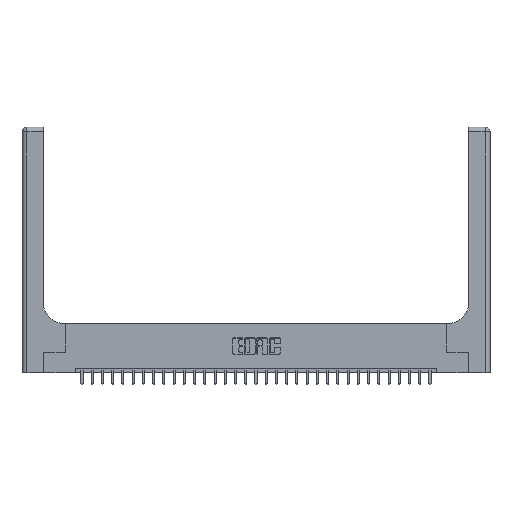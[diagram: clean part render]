
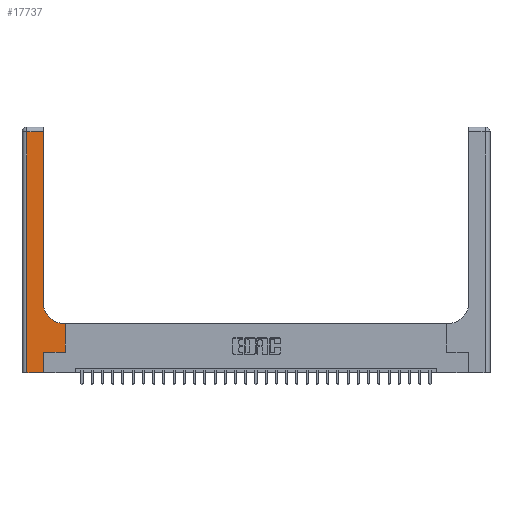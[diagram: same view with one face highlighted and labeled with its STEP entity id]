
A CAD part, top view. The second image highlights one B-rep face of the part: STEP entity #17737.
In plain terms, the highlighted planar face has unit normal (0, 0, 1).
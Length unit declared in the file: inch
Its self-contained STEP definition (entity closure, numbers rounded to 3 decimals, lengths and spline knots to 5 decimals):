
#203 = DIRECTION ( 'NONE',  ( 0., 0., -1. ) ) ;
#1018 = ORIENTED_EDGE ( 'NONE', *, *, #15994, .T. ) ;
#1087 = DIRECTION ( 'NONE',  ( 0., 1., 0. ) ) ;
#2089 = LINE ( 'NONE', #12986, #9763 ) ;
#2160 = EDGE_CURVE ( 'NONE', #9387, #17589, #18202, .T. ) ;
#2320 = ORIENTED_EDGE ( 'NONE', *, *, #22164, .T. ) ;
#2910 = CARTESIAN_POINT ( 'NONE',  ( 0.528, 0.6, 0.37 ) ) ;
#2916 = AXIS2_PLACEMENT_3D ( 'NONE', #20923, #203, #11976 ) ;
#2946 = CIRCLE ( 'NONE', #22953, 0.25 ) ;
#3421 = EDGE_CURVE ( 'NONE', #23773, #5509, #5814, .T. ) ;
#3538 = LINE ( 'NONE', #25630, #8011 ) ;
#3677 = VERTEX_POINT ( 'NONE', #5182 ) ;
#3708 = CARTESIAN_POINT ( 'NONE',  ( 0.528, 0.25, 0.37 ) ) ;
#4379 = CARTESIAN_POINT ( 'NONE',  ( 0.265, 0., 0.37 ) ) ;
#4380 = ORIENTED_EDGE ( 'NONE', *, *, #15150, .T. ) ;
#4567 = VERTEX_POINT ( 'NONE', #17945 ) ;
#4913 = DIRECTION ( 'NONE',  ( 1., 0., 0. ) ) ;
#5182 = CARTESIAN_POINT ( 'NONE',  ( 0.06, 2.94, 0.37 ) ) ;
#5497 = EDGE_CURVE ( 'NONE', #3677, #9387, #7105, .T. ) ;
#5509 = VERTEX_POINT ( 'NONE', #2910 ) ;
#5814 = LINE ( 'NONE', #3708, #28972 ) ;
#5893 = ORIENTED_EDGE ( 'NONE', *, *, #2160, .T. ) ;
#6213 = LINE ( 'NONE', #6357, #26730 ) ;
#6357 = CARTESIAN_POINT ( 'NONE',  ( 0., 2.94, 0.37 ) ) ;
#7105 = LINE ( 'NONE', #13254, #16096 ) ;
#7249 = DIRECTION ( 'NONE',  ( 0., -1., 0. ) ) ;
#7363 = CARTESIAN_POINT ( 'NONE',  ( 0.528, 0.25, 0.37 ) ) ;
#8011 = VECTOR ( 'NONE', #28156, 39.37008 ) ;
#8025 = EDGE_CURVE ( 'NONE', #17589, #13931, #14653, .T. ) ;
#8221 = CARTESIAN_POINT ( 'NONE',  ( 0.26, 0.85, 0.37 ) ) ;
#8770 = ORIENTED_EDGE ( 'NONE', *, *, #25700, .T. ) ;
#9369 = ORIENTED_EDGE ( 'NONE', *, *, #5497, .T. ) ;
#9387 = VERTEX_POINT ( 'NONE', #14657 ) ;
#9763 = VECTOR ( 'NONE', #26718, 39.37008 ) ;
#10508 = VECTOR ( 'NONE', #27422, 39.37008 ) ;
#11076 = CARTESIAN_POINT ( 'NONE',  ( 0.265, 0.25, 0.37 ) ) ;
#11976 = DIRECTION ( 'NONE',  ( -1., 0., 0. ) ) ;
#12208 = CARTESIAN_POINT ( 'NONE',  ( 0.265, 0.25, 0.37 ) ) ;
#12727 = EDGE_CURVE ( 'NONE', #5509, #17659, #3538, .T. ) ;
#12986 = CARTESIAN_POINT ( 'NONE',  ( 0.26, 3., 0.37 ) ) ;
#13254 = CARTESIAN_POINT ( 'NONE',  ( 0.06, 3., 0.37 ) ) ;
#13765 = PLANE ( 'NONE',  #2916 ) ;
#13871 = CARTESIAN_POINT ( 'NONE',  ( 0., 0., 0.37 ) ) ;
#13931 = VERTEX_POINT ( 'NONE', #11076 ) ;
#14653 = LINE ( 'NONE', #28355, #16477 ) ;
#14657 = CARTESIAN_POINT ( 'NONE',  ( 0.06, 0., 0.37 ) ) ;
#15123 = CARTESIAN_POINT ( 'NONE',  ( 0.51, 0.85, 0.37 ) ) ;
#15150 = EDGE_CURVE ( 'NONE', #13931, #23773, #23411, .T. ) ;
#15439 = DIRECTION ( 'NONE',  ( -1., 0., 0. ) ) ;
#15694 = ORIENTED_EDGE ( 'NONE', *, *, #3421, .T. ) ;
#15994 = EDGE_CURVE ( 'NONE', #4567, #3677, #6213, .T. ) ;
#16096 = VECTOR ( 'NONE', #7249, 39.37008 ) ;
#16477 = VECTOR ( 'NONE', #1087, 39.37008 ) ;
#17589 = VERTEX_POINT ( 'NONE', #4379 ) ;
#17659 = VERTEX_POINT ( 'NONE', #28981 ) ;
#17737 = ADVANCED_FACE ( 'NONE', ( #20491 ), #13765, .F. ) ;
#17945 = CARTESIAN_POINT ( 'NONE',  ( 0.26, 2.94, 0.37 ) ) ;
#18202 = LINE ( 'NONE', #13871, #22926 ) ;
#19459 = DIRECTION ( 'NONE',  ( 1., 0., 0. ) ) ;
#20491 = FACE_OUTER_BOUND ( 'NONE', #23975, .T. ) ;
#20923 = CARTESIAN_POINT ( 'NONE',  ( 0., 3., 0.37 ) ) ;
#22164 = EDGE_CURVE ( 'NONE', #17659, #29156, #2946, .T. ) ;
#22926 = VECTOR ( 'NONE', #4913, 39.37008 ) ;
#22953 = AXIS2_PLACEMENT_3D ( 'NONE', #15123, #28980, #19459 ) ;
#23411 = LINE ( 'NONE', #12208, #10508 ) ;
#23773 = VERTEX_POINT ( 'NONE', #7363 ) ;
#23975 = EDGE_LOOP ( 'NONE', ( #8770, #1018, #9369, #5893, #26612, #4380, #15694, #25090, #2320 ) ) ;
#23996 = DIRECTION ( 'NONE',  ( 0., 1., 0. ) ) ;
#25090 = ORIENTED_EDGE ( 'NONE', *, *, #12727, .T. ) ;
#25630 = CARTESIAN_POINT ( 'NONE',  ( 0.26, 0.6, 0.37 ) ) ;
#25700 = EDGE_CURVE ( 'NONE', #29156, #4567, #2089, .T. ) ;
#26612 = ORIENTED_EDGE ( 'NONE', *, *, #8025, .T. ) ;
#26718 = DIRECTION ( 'NONE',  ( 0., 1., 0. ) ) ;
#26730 = VECTOR ( 'NONE', #15439, 39.37008 ) ;
#27422 = DIRECTION ( 'NONE',  ( 1., 0., 0. ) ) ;
#28156 = DIRECTION ( 'NONE',  ( -1., 0., 0. ) ) ;
#28355 = CARTESIAN_POINT ( 'NONE',  ( 0.265, 0., 0.37 ) ) ;
#28972 = VECTOR ( 'NONE', #23996, 39.37008 ) ;
#28980 = DIRECTION ( 'NONE',  ( 0., 0., -1. ) ) ;
#28981 = CARTESIAN_POINT ( 'NONE',  ( 0.51, 0.6, 0.37 ) ) ;
#29156 = VERTEX_POINT ( 'NONE', #8221 ) ;
